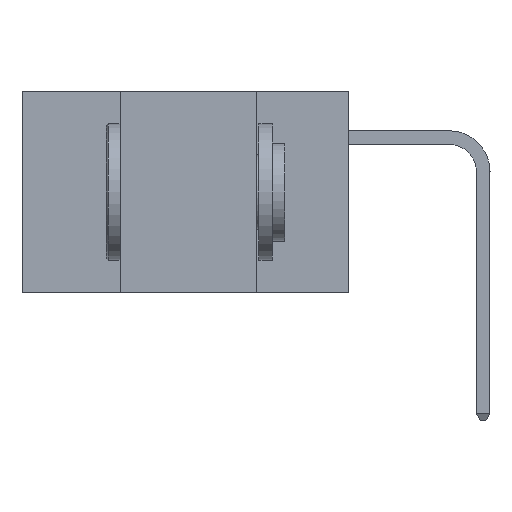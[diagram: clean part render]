
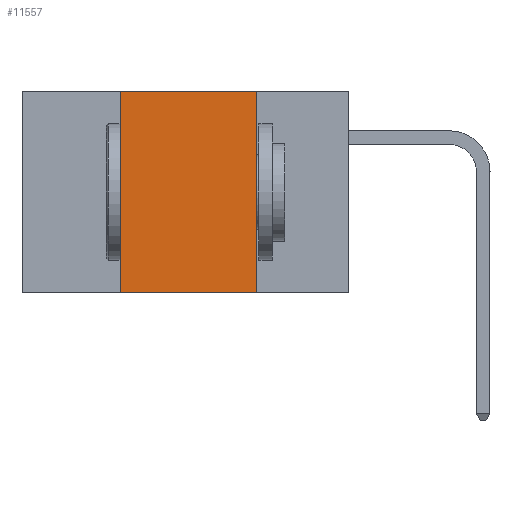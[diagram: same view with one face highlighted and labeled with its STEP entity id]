
A CAD part, left-side view. The second image highlights one B-rep face of the part: STEP entity #11557.
In plain terms, the highlighted planar face has unit normal (-1, 0, 0).
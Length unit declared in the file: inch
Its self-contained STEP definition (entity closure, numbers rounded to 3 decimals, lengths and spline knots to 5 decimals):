
#371 = ORIENTED_EDGE ( 'NONE', *, *, #29755, .F. ) ;
#459 = EDGE_CURVE ( 'NONE', #26926, #30646, #21540, .T. ) ;
#483 = PLANE ( 'NONE',  #19134 ) ;
#1264 = CARTESIAN_POINT ( 'NONE',  ( 0., 0.17, 0. ) ) ;
#2433 = CARTESIAN_POINT ( 'NONE',  ( 0., 0.6, -0.37 ) ) ;
#2619 = EDGE_LOOP ( 'NONE', ( #13044, #371, #8925, #3079 ) ) ;
#3079 = ORIENTED_EDGE ( 'NONE', *, *, #24360, .T. ) ;
#3235 = LINE ( 'NONE', #37008, #32932 ) ;
#3386 = DIRECTION ( 'NONE',  ( 0., 0., -1. ) ) ;
#5783 = FACE_OUTER_BOUND ( 'NONE', #2619, .T. ) ;
#5999 = LINE ( 'NONE', #30124, #35674 ) ;
#8925 = ORIENTED_EDGE ( 'NONE', *, *, #459, .F. ) ;
#8931 = DIRECTION ( 'NONE',  ( 0., 0., 1. ) ) ;
#11557 = ADVANCED_FACE ( 'NONE', ( #5783 ), #483, .F. ) ;
#13044 = ORIENTED_EDGE ( 'NONE', *, *, #27495, .F. ) ;
#13925 = VECTOR ( 'NONE', #8931, 39.37008 ) ;
#13986 = DIRECTION ( 'NONE',  ( 0., -1., 0. ) ) ;
#14355 = CARTESIAN_POINT ( 'NONE',  ( 0., 0.17, -0.37 ) ) ;
#16251 = LINE ( 'NONE', #2433, #37282 ) ;
#17878 = VERTEX_POINT ( 'NONE', #14355 ) ;
#19134 = AXIS2_PLACEMENT_3D ( 'NONE', #29214, #20660, #3386 ) ;
#20660 = DIRECTION ( 'NONE',  ( 1., 0., 0. ) ) ;
#21540 = LINE ( 'NONE', #32411, #13925 ) ;
#22905 = DIRECTION ( 'NONE',  ( 0., -1., 0. ) ) ;
#24360 = EDGE_CURVE ( 'NONE', #26926, #17878, #16251, .T. ) ;
#24597 = DIRECTION ( 'NONE',  ( 0., 0., -1. ) ) ;
#26926 = VERTEX_POINT ( 'NONE', #36387 ) ;
#27495 = EDGE_CURVE ( 'NONE', #36161, #17878, #5999, .T. ) ;
#29214 = CARTESIAN_POINT ( 'NONE',  ( 0., 0.6, 0. ) ) ;
#29739 = CARTESIAN_POINT ( 'NONE',  ( 0., 0.42, 0. ) ) ;
#29755 = EDGE_CURVE ( 'NONE', #30646, #36161, #3235, .T. ) ;
#30124 = CARTESIAN_POINT ( 'NONE',  ( 0., 0.17, 0. ) ) ;
#30646 = VERTEX_POINT ( 'NONE', #29739 ) ;
#32411 = CARTESIAN_POINT ( 'NONE',  ( 0., 0.42, 0. ) ) ;
#32932 = VECTOR ( 'NONE', #22905, 39.37008 ) ;
#35674 = VECTOR ( 'NONE', #24597, 39.37008 ) ;
#36161 = VERTEX_POINT ( 'NONE', #1264 ) ;
#36387 = CARTESIAN_POINT ( 'NONE',  ( 0., 0.42, -0.37 ) ) ;
#37008 = CARTESIAN_POINT ( 'NONE',  ( 0., 0.6, 0. ) ) ;
#37282 = VECTOR ( 'NONE', #13986, 39.37008 ) ;
